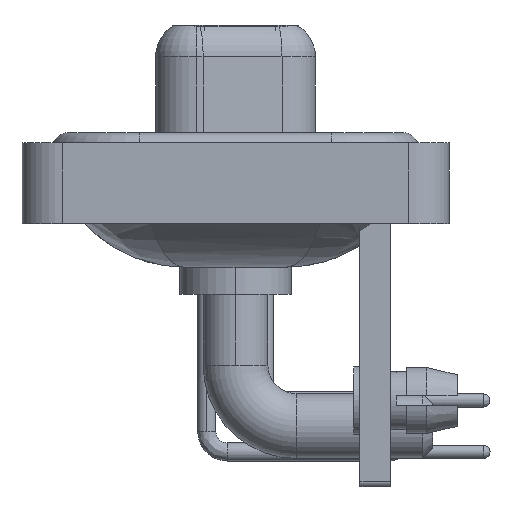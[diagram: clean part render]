
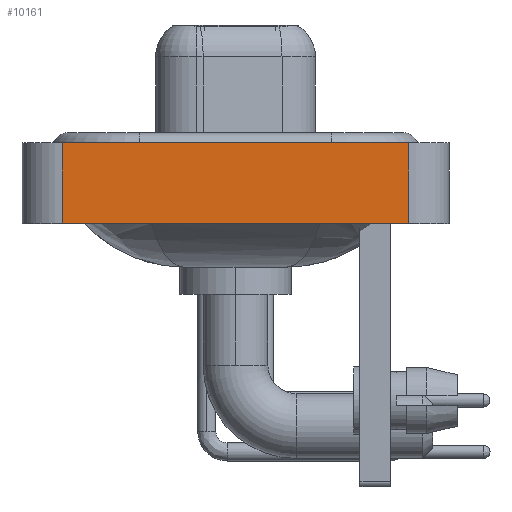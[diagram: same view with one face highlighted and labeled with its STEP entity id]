
A CAD part, left-side view. The second image highlights one B-rep face of the part: STEP entity #10161.
In plain terms, the highlighted planar face has unit normal (-1, 0, 0).
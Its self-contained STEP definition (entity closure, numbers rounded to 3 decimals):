
#1649 = LINE ( 'NONE', #24766, #11451 ) ;
#2902 = CARTESIAN_POINT ( 'NONE',  ( -7.35, -8.55, -3.6 ) ) ;
#3503 = VERTEX_POINT ( 'NONE', #14836 ) ;
#3750 = ORIENTED_EDGE ( 'NONE', *, *, #20013, .T. ) ;
#6129 = VERTEX_POINT ( 'NONE', #6977 ) ;
#6977 = CARTESIAN_POINT ( 'NONE',  ( -7.35, -8.55, 0.4 ) ) ;
#8080 = ORIENTED_EDGE ( 'NONE', *, *, #25730, .T. ) ;
#8703 = PLANE ( 'NONE',  #18219 ) ;
#8832 = CARTESIAN_POINT ( 'NONE',  ( -7.35, -8.55, -3.6 ) ) ;
#10161 = ADVANCED_FACE ( 'NONE', ( #10472 ), #8703, .T. ) ;
#10472 = FACE_OUTER_BOUND ( 'NONE', #17747, .T. ) ;
#10736 = EDGE_CURVE ( 'NONE', #21226, #3503, #17405, .T. ) ;
#11425 = DIRECTION ( 'NONE',  ( 0., 0., 1. ) ) ;
#11451 = VECTOR ( 'NONE', #26689, 1000. ) ;
#12235 = LINE ( 'NONE', #16309, #15174 ) ;
#12306 = CARTESIAN_POINT ( 'NONE',  ( -7.35, -8.55, 0.4 ) ) ;
#12570 = ORIENTED_EDGE ( 'NONE', *, *, #10736, .F. ) ;
#14308 = EDGE_CURVE ( 'NONE', #3503, #6129, #16384, .T. ) ;
#14836 = CARTESIAN_POINT ( 'NONE',  ( -7.35, 8.55, 0.4 ) ) ;
#15114 = DIRECTION ( 'NONE',  ( -1., 0., 0. ) ) ;
#15174 = VECTOR ( 'NONE', #24682, 1000. ) ;
#15501 = CARTESIAN_POINT ( 'NONE',  ( -7.35, 8.55, -3.6 ) ) ;
#16309 = CARTESIAN_POINT ( 'NONE',  ( -7.35, -8.55, -3.6 ) ) ;
#16384 = LINE ( 'NONE', #12306, #23539 ) ;
#16613 = VERTEX_POINT ( 'NONE', #2902 ) ;
#17405 = LINE ( 'NONE', #15501, #24758 ) ;
#17747 = EDGE_LOOP ( 'NONE', ( #3750, #23872, #12570, #8080 ) ) ;
#18219 = AXIS2_PLACEMENT_3D ( 'NONE', #8832, #15114, #21135 ) ;
#20013 = EDGE_CURVE ( 'NONE', #16613, #6129, #12235, .T. ) ;
#20634 = DIRECTION ( 'NONE',  ( 0., -1., 0. ) ) ;
#21135 = DIRECTION ( 'NONE',  ( 0., 0., 1. ) ) ;
#21226 = VERTEX_POINT ( 'NONE', #21922 ) ;
#21922 = CARTESIAN_POINT ( 'NONE',  ( -7.35, 8.55, -3.6 ) ) ;
#23539 = VECTOR ( 'NONE', #20634, 1000. ) ;
#23872 = ORIENTED_EDGE ( 'NONE', *, *, #14308, .F. ) ;
#24682 = DIRECTION ( 'NONE',  ( 0., 0., 1. ) ) ;
#24758 = VECTOR ( 'NONE', #11425, 1000. ) ;
#24766 = CARTESIAN_POINT ( 'NONE',  ( -7.35, -8.55, -3.6 ) ) ;
#25730 = EDGE_CURVE ( 'NONE', #21226, #16613, #1649, .T. ) ;
#26689 = DIRECTION ( 'NONE',  ( 0., -1., 0. ) ) ;
